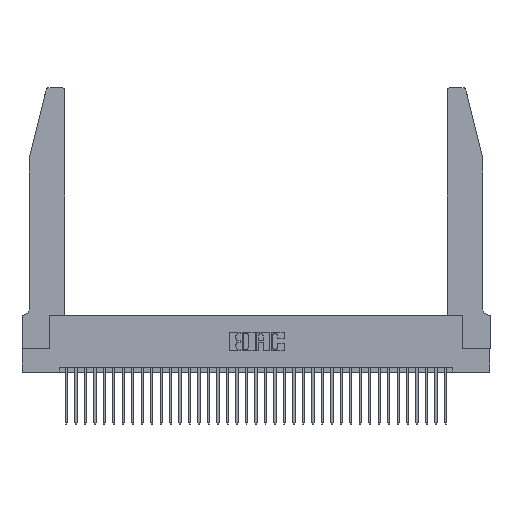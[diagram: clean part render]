
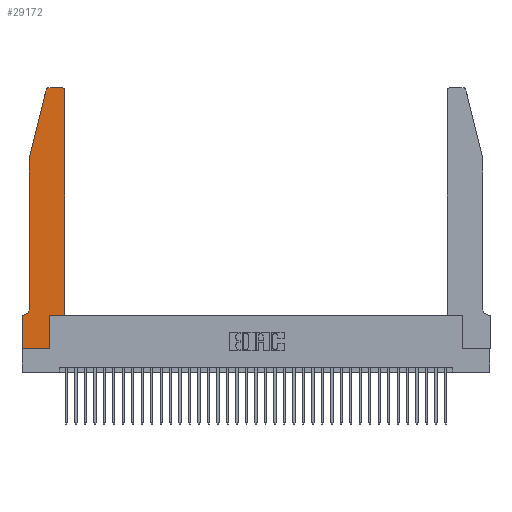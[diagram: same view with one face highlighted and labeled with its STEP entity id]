
A CAD part, top view. The second image highlights one B-rep face of the part: STEP entity #29172.
In plain terms, the highlighted planar face has unit normal (0, 0, 1).
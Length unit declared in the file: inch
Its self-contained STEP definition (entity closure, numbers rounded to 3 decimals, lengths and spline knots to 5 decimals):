
#145 = VECTOR ( 'NONE', #35649, 39.37008 ) ;
#227 = VECTOR ( 'NONE', #36706, 39.37008 ) ;
#1640 = CARTESIAN_POINT ( 'NONE',  ( 0.4505, 0.35, 0.37 ) ) ;
#2343 = EDGE_CURVE ( 'NONE', #4399, #16705, #7743, .T. ) ;
#3049 = VECTOR ( 'NONE', #3755, 39.37008 ) ;
#3215 = ORIENTED_EDGE ( 'NONE', *, *, #12529, .T. ) ;
#3508 = CARTESIAN_POINT ( 'NONE',  ( 0.0055, 0.42, 0.37 ) ) ;
#3755 = DIRECTION ( 'NONE',  ( 1., 0., 0. ) ) ;
#3784 = PLANE ( 'NONE',  #17751 ) ;
#4222 = EDGE_CURVE ( 'NONE', #21414, #4399, #29503, .T. ) ;
#4399 = VERTEX_POINT ( 'NONE', #32565 ) ;
#4472 = VERTEX_POINT ( 'NONE', #1640 ) ;
#4677 = DIRECTION ( 'NONE',  ( 0., -1., 0. ) ) ;
#5050 = DIRECTION ( 'NONE',  ( 0., 1., 0. ) ) ;
#5192 = CARTESIAN_POINT ( 'NONE',  ( 0.0755, 0.35, 0.37 ) ) ;
#5602 = CARTESIAN_POINT ( 'NONE',  ( 0.0755, 2., 0.37 ) ) ;
#5603 = CARTESIAN_POINT ( 'NONE',  ( 0.2605, 2.75, 0.37 ) ) ;
#5728 = EDGE_CURVE ( 'NONE', #24478, #21414, #25468, .T. ) ;
#5945 = ORIENTED_EDGE ( 'NONE', *, *, #33252, .T. ) ;
#6011 = VERTEX_POINT ( 'NONE', #35147 ) ;
#6443 = DIRECTION ( 'NONE',  ( -1., 0., 0. ) ) ;
#6685 = VECTOR ( 'NONE', #11478, 39.37008 ) ;
#7043 = LINE ( 'NONE', #15919, #145 ) ;
#7376 = VECTOR ( 'NONE', #5050, 39.37008 ) ;
#7743 = CIRCLE ( 'NONE', #34015, 0.03 ) ;
#7777 = ORIENTED_EDGE ( 'NONE', *, *, #29732, .T. ) ;
#8826 = CARTESIAN_POINT ( 'NONE',  ( 0.4505, 2.72, 0.37 ) ) ;
#8965 = LINE ( 'NONE', #36583, #227 ) ;
#9089 = CARTESIAN_POINT ( 'NONE',  ( 0.0755, 2., 0.37 ) ) ;
#9628 = ORIENTED_EDGE ( 'NONE', *, *, #10492, .T. ) ;
#10185 = VECTOR ( 'NONE', #18645, 39.37008 ) ;
#10492 = EDGE_CURVE ( 'NONE', #13019, #16172, #8965, .T. ) ;
#10980 = ORIENTED_EDGE ( 'NONE', *, *, #21107, .T. ) ;
#11446 = ORIENTED_EDGE ( 'NONE', *, *, #22917, .T. ) ;
#11478 = DIRECTION ( 'NONE',  ( -1., 0., 0. ) ) ;
#11752 = AXIS2_PLACEMENT_3D ( 'NONE', #14268, #34038, #17167 ) ;
#11997 = DIRECTION ( 'NONE',  ( 0., -1., 0. ) ) ;
#12183 = VERTEX_POINT ( 'NONE', #5602 ) ;
#12362 = DIRECTION ( 'NONE',  ( 0., 0., 1. ) ) ;
#12459 = DIRECTION ( 'NONE',  ( 0., 0., 1. ) ) ;
#12529 = EDGE_CURVE ( 'NONE', #16705, #12183, #25351, .T. ) ;
#12562 = CARTESIAN_POINT ( 'NONE',  ( 0., 0., 0.37 ) ) ;
#13019 = VERTEX_POINT ( 'NONE', #21160 ) ;
#13198 = CARTESIAN_POINT ( 'NONE',  ( 0., 0., 0.37 ) ) ;
#13735 = ORIENTED_EDGE ( 'NONE', *, *, #19415, .T. ) ;
#14137 = ORIENTED_EDGE ( 'NONE', *, *, #4222, .T. ) ;
#14268 = CARTESIAN_POINT ( 'NONE',  ( 0.4205, 2.72, 0.37 ) ) ;
#15919 = CARTESIAN_POINT ( 'NONE',  ( 0.4505, 0.35, 0.37 ) ) ;
#16172 = VERTEX_POINT ( 'NONE', #19753 ) ;
#16705 = VERTEX_POINT ( 'NONE', #24893 ) ;
#16765 = EDGE_CURVE ( 'NONE', #4472, #24478, #36756, .T. ) ;
#16779 = DIRECTION ( 'NONE',  ( -1., 0., 0. ) ) ;
#17167 = DIRECTION ( 'NONE',  ( 1., 0., 0. ) ) ;
#17402 = CARTESIAN_POINT ( 'NONE',  ( 0.0055, 0.35, 0.37 ) ) ;
#17751 = AXIS2_PLACEMENT_3D ( 'NONE', #18258, #12459, #23919 ) ;
#18258 = CARTESIAN_POINT ( 'NONE',  ( 0., 0.35, 0.37 ) ) ;
#18645 = DIRECTION ( 'NONE',  ( -0.239, -0.971, 0. ) ) ;
#19415 = EDGE_CURVE ( 'NONE', #6011, #23692, #34853, .T. ) ;
#19753 = CARTESIAN_POINT ( 'NONE',  ( 0.2865, 0.35, 0.37 ) ) ;
#21067 = VECTOR ( 'NONE', #11997, 39.37008 ) ;
#21107 = EDGE_CURVE ( 'NONE', #12183, #35691, #35195, .T. ) ;
#21160 = CARTESIAN_POINT ( 'NONE',  ( 0.2865, 0., 0.37 ) ) ;
#21414 = VERTEX_POINT ( 'NONE', #27540 ) ;
#22372 = EDGE_CURVE ( 'NONE', #35691, #25998, #25013, .T. ) ;
#22917 = EDGE_CURVE ( 'NONE', #16172, #4472, #7043, .T. ) ;
#23483 = ORIENTED_EDGE ( 'NONE', *, *, #2343, .T. ) ;
#23648 = DIRECTION ( 'NONE',  ( 0., 0., -1. ) ) ;
#23692 = VERTEX_POINT ( 'NONE', #13198 ) ;
#23833 = CARTESIAN_POINT ( 'NONE',  ( 0.0755, 0.42, 0.37 ) ) ;
#23919 = DIRECTION ( 'NONE',  ( 1., 0., 0. ) ) ;
#24203 = LINE ( 'NONE', #12562, #3049 ) ;
#24478 = VERTEX_POINT ( 'NONE', #8826 ) ;
#24777 = CARTESIAN_POINT ( 'NONE',  ( 0., 0., 0.37 ) ) ;
#24893 = CARTESIAN_POINT ( 'NONE',  ( 0.25487, 2.72718, 0.37 ) ) ;
#25013 = CIRCLE ( 'NONE', #29412, 0.07 ) ;
#25147 = CARTESIAN_POINT ( 'NONE',  ( 0.4505, 0.35, 0.37 ) ) ;
#25351 = LINE ( 'NONE', #29987, #10185 ) ;
#25468 = CIRCLE ( 'NONE', #11752, 0.03 ) ;
#25998 = VERTEX_POINT ( 'NONE', #17402 ) ;
#26483 = VECTOR ( 'NONE', #4677, 39.37008 ) ;
#26514 = VECTOR ( 'NONE', #16779, 39.37008 ) ;
#26594 = ORIENTED_EDGE ( 'NONE', *, *, #16765, .T. ) ;
#27540 = CARTESIAN_POINT ( 'NONE',  ( 0.4205, 2.75, 0.37 ) ) ;
#29172 = ADVANCED_FACE ( 'NONE', ( #35264 ), #3784, .T. ) ;
#29383 = CARTESIAN_POINT ( 'NONE',  ( 0.284, 2.72, 0.37 ) ) ;
#29412 = AXIS2_PLACEMENT_3D ( 'NONE', #3508, #23648, #6443 ) ;
#29503 = LINE ( 'NONE', #5603, #6685 ) ;
#29732 = EDGE_CURVE ( 'NONE', #23692, #13019, #24203, .T. ) ;
#29987 = CARTESIAN_POINT ( 'NONE',  ( 0.0755, 2., 0.37 ) ) ;
#30592 = EDGE_LOOP ( 'NONE', ( #14137, #23483, #3215, #10980, #35399, #5945, #13735, #7777, #9628, #11446, #26594, #34065 ) ) ;
#32206 = DIRECTION ( 'NONE',  ( 1., 0., 0. ) ) ;
#32565 = CARTESIAN_POINT ( 'NONE',  ( 0.284, 2.75, 0.37 ) ) ;
#33100 = LINE ( 'NONE', #5192, #26514 ) ;
#33252 = EDGE_CURVE ( 'NONE', #25998, #6011, #33100, .T. ) ;
#34015 = AXIS2_PLACEMENT_3D ( 'NONE', #29383, #12362, #32206 ) ;
#34038 = DIRECTION ( 'NONE',  ( 0., 0., 1. ) ) ;
#34065 = ORIENTED_EDGE ( 'NONE', *, *, #5728, .T. ) ;
#34853 = LINE ( 'NONE', #24777, #26483 ) ;
#35147 = CARTESIAN_POINT ( 'NONE',  ( 0., 0.35, 0.37 ) ) ;
#35195 = LINE ( 'NONE', #9089, #21067 ) ;
#35264 = FACE_OUTER_BOUND ( 'NONE', #30592, .T. ) ;
#35399 = ORIENTED_EDGE ( 'NONE', *, *, #22372, .T. ) ;
#35649 = DIRECTION ( 'NONE',  ( 1., 0., 0. ) ) ;
#35691 = VERTEX_POINT ( 'NONE', #23833 ) ;
#36583 = CARTESIAN_POINT ( 'NONE',  ( 0.2865, 0.35, 0.37 ) ) ;
#36706 = DIRECTION ( 'NONE',  ( 0., 1., 0. ) ) ;
#36756 = LINE ( 'NONE', #25147, #7376 ) ;
